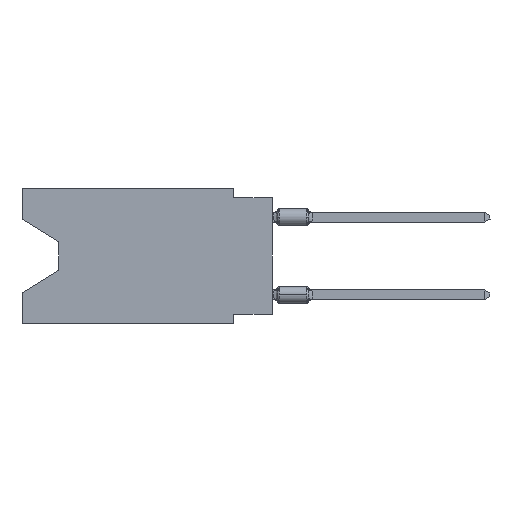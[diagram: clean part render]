
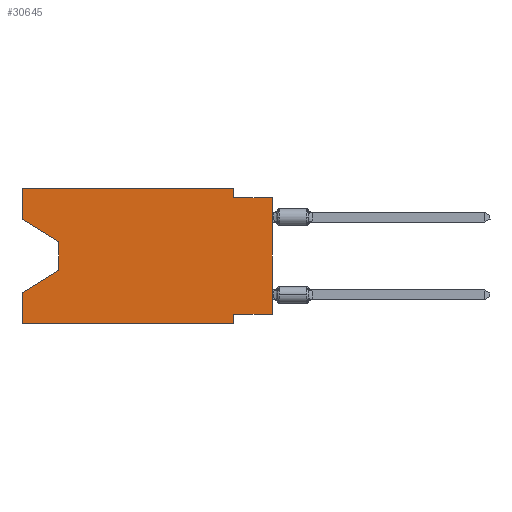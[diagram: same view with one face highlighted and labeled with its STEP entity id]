
A CAD part, left-side view. The second image highlights one B-rep face of the part: STEP entity #30645.
In plain terms, the highlighted planar face has unit normal (-1, 0, 0).
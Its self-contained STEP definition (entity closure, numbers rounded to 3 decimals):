
#27 = CARTESIAN_POINT ( 'NONE',  ( 0., 2.54, -8.89 ) ) ;
#738 = CARTESIAN_POINT ( 'NONE',  ( 0., 13.97, -3.505 ) ) ;
#851 = DIRECTION ( 'NONE',  ( 0., 0., 1. ) ) ;
#1142 = LINE ( 'NONE', #35808, #8857 ) ;
#1353 = DIRECTION ( 'NONE',  ( 0., 0.855, -0.519 ) ) ;
#1943 = EDGE_CURVE ( 'NONE', #15668, #21356, #23462, .T. ) ;
#3151 = CARTESIAN_POINT ( 'NONE',  ( 0., 2.54, -0.635 ) ) ;
#3500 = ORIENTED_EDGE ( 'NONE', *, *, #12586, .T. ) ;
#4180 = VERTEX_POINT ( 'NONE', #27 ) ;
#4800 = VERTEX_POINT ( 'NONE', #738 ) ;
#5743 = LINE ( 'NONE', #22767, #36347 ) ;
#5757 = CARTESIAN_POINT ( 'NONE',  ( 0., 16.383, -8.89 ) ) ;
#5786 = EDGE_CURVE ( 'NONE', #21052, #15668, #19749, .T. ) ;
#7068 = CARTESIAN_POINT ( 'NONE',  ( 0., 16.383, -2.038 ) ) ;
#8260 = ORIENTED_EDGE ( 'NONE', *, *, #22528, .F. ) ;
#8349 = VECTOR ( 'NONE', #20381, 1000. ) ;
#8550 = DIRECTION ( 'NONE',  ( 0., 0., -1. ) ) ;
#8717 = DIRECTION ( 'NONE',  ( 0., 0., -1. ) ) ;
#8857 = VECTOR ( 'NONE', #12938, 1000. ) ;
#9081 = VECTOR ( 'NONE', #851, 1000. ) ;
#9399 = CARTESIAN_POINT ( 'NONE',  ( 0., 2.54, -8.89 ) ) ;
#10565 = CARTESIAN_POINT ( 'NONE',  ( 0., 16.383, -8.89 ) ) ;
#10836 = VECTOR ( 'NONE', #35886, 1000. ) ;
#11506 = ORIENTED_EDGE ( 'NONE', *, *, #31088, .T. ) ;
#11968 = VERTEX_POINT ( 'NONE', #30112 ) ;
#12078 = EDGE_CURVE ( 'NONE', #29953, #4180, #37090, .T. ) ;
#12586 = EDGE_CURVE ( 'NONE', #4800, #11968, #20722, .T. ) ;
#12938 = DIRECTION ( 'NONE',  ( 0., -1., 0. ) ) ;
#13657 = ORIENTED_EDGE ( 'NONE', *, *, #19582, .T. ) ;
#13801 = ORIENTED_EDGE ( 'NONE', *, *, #31897, .F. ) ;
#14132 = ORIENTED_EDGE ( 'NONE', *, *, #5786, .F. ) ;
#14356 = CARTESIAN_POINT ( 'NONE',  ( 0., 0., -0.635 ) ) ;
#15668 = VERTEX_POINT ( 'NONE', #3151 ) ;
#16180 = DIRECTION ( 'NONE',  ( 0., -1., 0. ) ) ;
#16297 = CARTESIAN_POINT ( 'NONE',  ( 0., 0., -0.635 ) ) ;
#16609 = ORIENTED_EDGE ( 'NONE', *, *, #12078, .T. ) ;
#16746 = EDGE_CURVE ( 'NONE', #18903, #33146, #28494, .T. ) ;
#16830 = DIRECTION ( 'NONE',  ( 0., 0., -1. ) ) ;
#17229 = VECTOR ( 'NONE', #16180, 1000. ) ;
#18903 = VERTEX_POINT ( 'NONE', #7068 ) ;
#18929 = VECTOR ( 'NONE', #8717, 1000. ) ;
#19036 = LINE ( 'NONE', #36266, #9081 ) ;
#19167 = CARTESIAN_POINT ( 'NONE',  ( 0., 13.97, -5.385 ) ) ;
#19315 = VECTOR ( 'NONE', #16830, 1000. ) ;
#19582 = EDGE_CURVE ( 'NONE', #18903, #4800, #5743, .T. ) ;
#19708 = EDGE_LOOP ( 'NONE', ( #13657, #3500, #23427, #27968, #16609, #8260, #25076, #11506, #28767, #14132, #13801, #32466 ) ) ;
#19749 = LINE ( 'NONE', #31538, #19315 ) ;
#20176 = PLANE ( 'NONE',  #23275 ) ;
#20381 = DIRECTION ( 'NONE',  ( 0., 0., 1. ) ) ;
#20599 = CARTESIAN_POINT ( 'NONE',  ( 0., 0., -8.255 ) ) ;
#20722 = LINE ( 'NONE', #24183, #18929 ) ;
#21052 = VERTEX_POINT ( 'NONE', #23102 ) ;
#21356 = VERTEX_POINT ( 'NONE', #16297 ) ;
#22156 = CARTESIAN_POINT ( 'NONE',  ( 0., 2.54, -8.255 ) ) ;
#22528 = EDGE_CURVE ( 'NONE', #26065, #4180, #30466, .T. ) ;
#22767 = CARTESIAN_POINT ( 'NONE',  ( 0., 16.383, -2.038 ) ) ;
#22884 = DIRECTION ( 'NONE',  ( 1., 0., 0. ) ) ;
#23011 = CARTESIAN_POINT ( 'NONE',  ( 0., 0., -8.255 ) ) ;
#23102 = CARTESIAN_POINT ( 'NONE',  ( 0., 2.54, 0. ) ) ;
#23139 = VECTOR ( 'NONE', #1353, 1000. ) ;
#23275 = AXIS2_PLACEMENT_3D ( 'NONE', #35068, #22884, #8550 ) ;
#23427 = ORIENTED_EDGE ( 'NONE', *, *, #26429, .T. ) ;
#23462 = LINE ( 'NONE', #14356, #24059 ) ;
#24059 = VECTOR ( 'NONE', #34504, 1000. ) ;
#24183 = CARTESIAN_POINT ( 'NONE',  ( 0., 13.97, -3.505 ) ) ;
#25076 = ORIENTED_EDGE ( 'NONE', *, *, #29210, .F. ) ;
#26065 = VERTEX_POINT ( 'NONE', #22156 ) ;
#26167 = CARTESIAN_POINT ( 'NONE',  ( 0., 16.383, 0. ) ) ;
#26429 = EDGE_CURVE ( 'NONE', #11968, #28015, #37149, .T. ) ;
#26589 = LINE ( 'NONE', #20599, #10836 ) ;
#27646 = CARTESIAN_POINT ( 'NONE',  ( 0., 16.383, 0. ) ) ;
#27968 = ORIENTED_EDGE ( 'NONE', *, *, #32917, .F. ) ;
#28015 = VERTEX_POINT ( 'NONE', #29982 ) ;
#28494 = LINE ( 'NONE', #26167, #8349 ) ;
#28663 = FACE_OUTER_BOUND ( 'NONE', #19708, .T. ) ;
#28767 = ORIENTED_EDGE ( 'NONE', *, *, #1943, .F. ) ;
#29210 = EDGE_CURVE ( 'NONE', #29636, #26065, #26589, .T. ) ;
#29636 = VERTEX_POINT ( 'NONE', #23011 ) ;
#29953 = VERTEX_POINT ( 'NONE', #5757 ) ;
#29982 = CARTESIAN_POINT ( 'NONE',  ( 0., 16.383, -6.852 ) ) ;
#30112 = CARTESIAN_POINT ( 'NONE',  ( 0., 13.97, -5.385 ) ) ;
#30466 = LINE ( 'NONE', #9399, #34550 ) ;
#30645 = ADVANCED_FACE ( 'NONE', ( #28663 ), #20176, .F. ) ;
#31072 = VECTOR ( 'NONE', #32514, 1000. ) ;
#31088 = EDGE_CURVE ( 'NONE', #29636, #21356, #19036, .T. ) ;
#31473 = DIRECTION ( 'NONE',  ( 0., -0.855, -0.519 ) ) ;
#31538 = CARTESIAN_POINT ( 'NONE',  ( 0., 2.54, 0. ) ) ;
#31897 = EDGE_CURVE ( 'NONE', #33146, #21052, #1142, .T. ) ;
#32466 = ORIENTED_EDGE ( 'NONE', *, *, #16746, .F. ) ;
#32514 = DIRECTION ( 'NONE',  ( 0., 0., 1. ) ) ;
#32917 = EDGE_CURVE ( 'NONE', #29953, #28015, #35036, .T. ) ;
#33146 = VERTEX_POINT ( 'NONE', #27646 ) ;
#33401 = DIRECTION ( 'NONE',  ( 0., 0., -1. ) ) ;
#34504 = DIRECTION ( 'NONE',  ( 0., -1., 0. ) ) ;
#34550 = VECTOR ( 'NONE', #33401, 1000. ) ;
#35036 = LINE ( 'NONE', #37941, #31072 ) ;
#35068 = CARTESIAN_POINT ( 'NONE',  ( 0., 16.383, 0. ) ) ;
#35808 = CARTESIAN_POINT ( 'NONE',  ( 0., 16.383, 0. ) ) ;
#35886 = DIRECTION ( 'NONE',  ( 0., 1., 0. ) ) ;
#36266 = CARTESIAN_POINT ( 'NONE',  ( 0., 0., 0. ) ) ;
#36347 = VECTOR ( 'NONE', #31473, 1000. ) ;
#37090 = LINE ( 'NONE', #10565, #17229 ) ;
#37149 = LINE ( 'NONE', #19167, #23139 ) ;
#37941 = CARTESIAN_POINT ( 'NONE',  ( 0., 16.383, 0. ) ) ;
